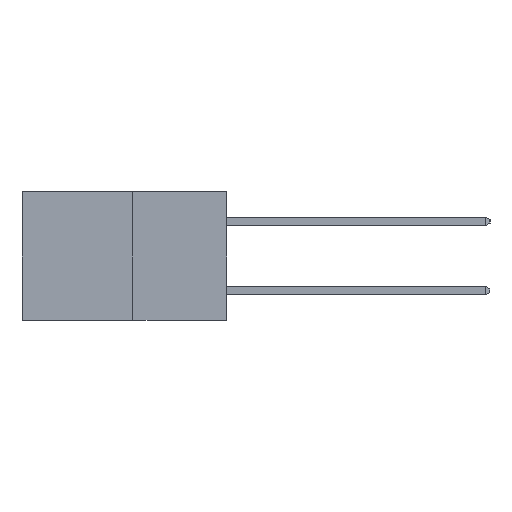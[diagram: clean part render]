
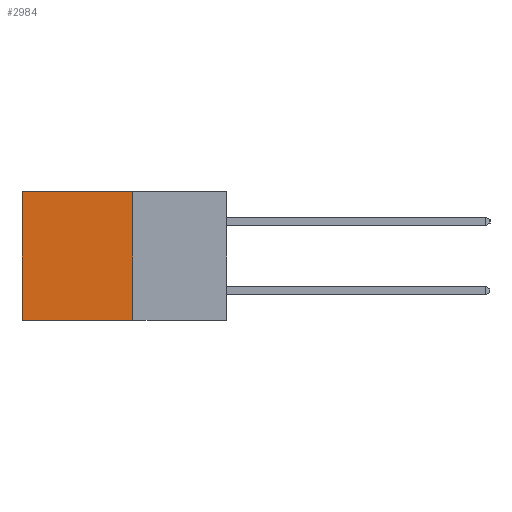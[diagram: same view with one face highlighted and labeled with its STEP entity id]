
A CAD part, left-side view. The second image highlights one B-rep face of the part: STEP entity #2984.
In plain terms, the highlighted planar face has unit normal (-1, 0, 0).
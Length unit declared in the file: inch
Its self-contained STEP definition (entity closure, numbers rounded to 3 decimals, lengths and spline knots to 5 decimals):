
#29 = CARTESIAN_POINT ( 'NONE',  ( 0.277, 0.27, 0. ) ) ;
#1468 = EDGE_CURVE ( 'NONE', #9786, #3042, #13636, .T. ) ;
#2666 = CARTESIAN_POINT ( 'NONE',  ( 0.277, 0.27, -0.37 ) ) ;
#2984 = ADVANCED_FACE ( 'NONE', ( #20276 ), #16012, .F. ) ;
#3042 = VERTEX_POINT ( 'NONE', #6928 ) ;
#3258 = VECTOR ( 'NONE', #5003, 39.37008 ) ;
#3451 = ORIENTED_EDGE ( 'NONE', *, *, #17364, .F. ) ;
#3790 = LINE ( 'NONE', #16802, #3258 ) ;
#4411 = DIRECTION ( 'NONE',  ( 0., 0., -1. ) ) ;
#5003 = DIRECTION ( 'NONE',  ( 0., 0., -1. ) ) ;
#6493 = VERTEX_POINT ( 'NONE', #13643 ) ;
#6497 = DIRECTION ( 'NONE',  ( 0., 1., 0. ) ) ;
#6647 = DIRECTION ( 'NONE',  ( 1., 0., 0. ) ) ;
#6928 = CARTESIAN_POINT ( 'NONE',  ( 0.277, 0.59, 0. ) ) ;
#7135 = CARTESIAN_POINT ( 'NONE',  ( 0.277, 0.59, -0.37 ) ) ;
#7484 = ORIENTED_EDGE ( 'NONE', *, *, #18124, .T. ) ;
#9006 = VERTEX_POINT ( 'NONE', #7135 ) ;
#9011 = DIRECTION ( 'NONE',  ( 0., 0., -1. ) ) ;
#9786 = VERTEX_POINT ( 'NONE', #10781 ) ;
#10694 = EDGE_LOOP ( 'NONE', ( #7484, #3451, #12509, #21290 ) ) ;
#10781 = CARTESIAN_POINT ( 'NONE',  ( 0.277, 0.27, 0. ) ) ;
#11226 = DIRECTION ( 'NONE',  ( 0., 1., 0. ) ) ;
#11712 = VECTOR ( 'NONE', #4411, 39.37008 ) ;
#12457 = EDGE_CURVE ( 'NONE', #9786, #6493, #20509, .T. ) ;
#12509 = ORIENTED_EDGE ( 'NONE', *, *, #12457, .F. ) ;
#13104 = VECTOR ( 'NONE', #6497, 39.37008 ) ;
#13636 = LINE ( 'NONE', #29, #13104 ) ;
#13643 = CARTESIAN_POINT ( 'NONE',  ( 0.277, 0.27, -0.37 ) ) ;
#14301 = AXIS2_PLACEMENT_3D ( 'NONE', #17535, #6647, #9011 ) ;
#16012 = PLANE ( 'NONE',  #14301 ) ;
#16802 = CARTESIAN_POINT ( 'NONE',  ( 0.277, 0.59, -0.37 ) ) ;
#17364 = EDGE_CURVE ( 'NONE', #6493, #9006, #20300, .T. ) ;
#17535 = CARTESIAN_POINT ( 'NONE',  ( 0.277, 0.27, -0.37 ) ) ;
#18124 = EDGE_CURVE ( 'NONE', #3042, #9006, #3790, .T. ) ;
#19488 = CARTESIAN_POINT ( 'NONE',  ( 0.277, 0.27, -0.37 ) ) ;
#20276 = FACE_OUTER_BOUND ( 'NONE', #10694, .T. ) ;
#20300 = LINE ( 'NONE', #19488, #20830 ) ;
#20509 = LINE ( 'NONE', #2666, #11712 ) ;
#20830 = VECTOR ( 'NONE', #11226, 39.37008 ) ;
#21290 = ORIENTED_EDGE ( 'NONE', *, *, #1468, .T. ) ;
